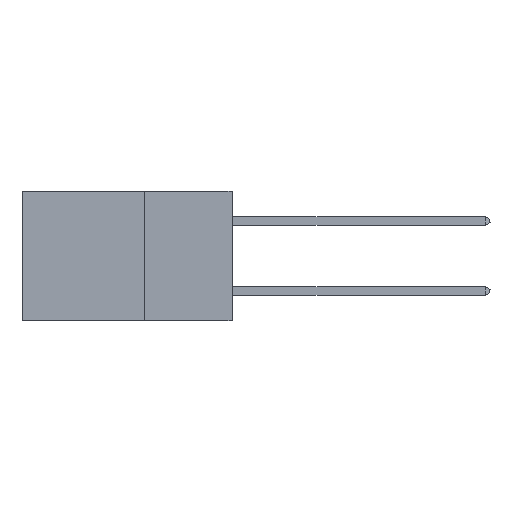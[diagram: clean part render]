
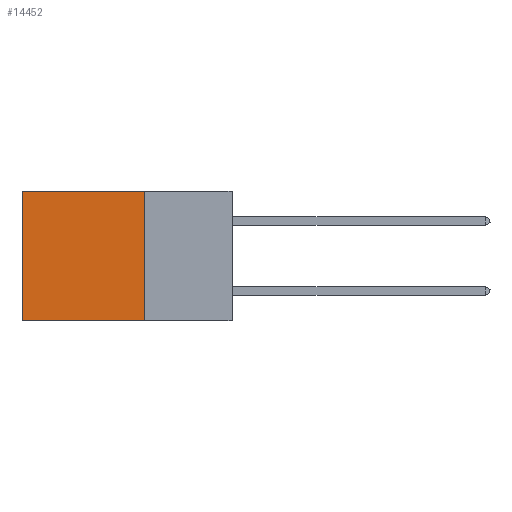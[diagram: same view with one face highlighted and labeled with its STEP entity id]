
A CAD part, left-side view. The second image highlights one B-rep face of the part: STEP entity #14452.
In plain terms, the highlighted planar face has unit normal (-1, 0, 0).
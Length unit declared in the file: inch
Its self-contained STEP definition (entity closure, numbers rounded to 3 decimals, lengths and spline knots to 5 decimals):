
#255 = VERTEX_POINT ( 'NONE', #7116 ) ;
#371 = LINE ( 'NONE', #24608, #9482 ) ;
#1425 = PLANE ( 'NONE',  #29148 ) ;
#1525 = ORIENTED_EDGE ( 'NONE', *, *, #15686, .F. ) ;
#3325 = CARTESIAN_POINT ( 'NONE',  ( 0.2875, 0.25, 0. ) ) ;
#4008 = DIRECTION ( 'NONE',  ( 0., 0., -1. ) ) ;
#5165 = CARTESIAN_POINT ( 'NONE',  ( 0.2875, 0.25, 0. ) ) ;
#5299 = VERTEX_POINT ( 'NONE', #12848 ) ;
#6133 = ORIENTED_EDGE ( 'NONE', *, *, #20132, .T. ) ;
#6477 = CARTESIAN_POINT ( 'NONE',  ( 0.2875, 0.25, -0.37 ) ) ;
#7116 = CARTESIAN_POINT ( 'NONE',  ( 0.2875, 0.25, 0. ) ) ;
#7707 = VERTEX_POINT ( 'NONE', #6477 ) ;
#7900 = DIRECTION ( 'NONE',  ( 0., 0., -1. ) ) ;
#8041 = DIRECTION ( 'NONE',  ( 0., 0., -1. ) ) ;
#8092 = ORIENTED_EDGE ( 'NONE', *, *, #29874, .F. ) ;
#9482 = VECTOR ( 'NONE', #32164, 39.37008 ) ;
#11299 = CARTESIAN_POINT ( 'NONE',  ( 0.2875, 0.6, -0.37 ) ) ;
#12848 = CARTESIAN_POINT ( 'NONE',  ( 0.2875, 0.6, 0. ) ) ;
#14452 = ADVANCED_FACE ( 'NONE', ( #27879 ), #1425, .F. ) ;
#15686 = EDGE_CURVE ( 'NONE', #7707, #18472, #371, .T. ) ;
#18472 = VERTEX_POINT ( 'NONE', #11299 ) ;
#19187 = DIRECTION ( 'NONE',  ( 1., 0., 0. ) ) ;
#20132 = EDGE_CURVE ( 'NONE', #5299, #18472, #22760, .T. ) ;
#20429 = LINE ( 'NONE', #3325, #23227 ) ;
#20488 = VECTOR ( 'NONE', #7900, 39.37008 ) ;
#20841 = CARTESIAN_POINT ( 'NONE',  ( 0.2875, 0.6, 0. ) ) ;
#21646 = ORIENTED_EDGE ( 'NONE', *, *, #30432, .T. ) ;
#22760 = LINE ( 'NONE', #20841, #24729 ) ;
#23227 = VECTOR ( 'NONE', #23855, 39.37008 ) ;
#23855 = DIRECTION ( 'NONE',  ( 0., 1., 0. ) ) ;
#24608 = CARTESIAN_POINT ( 'NONE',  ( 0.2875, 0.25, -0.37 ) ) ;
#24729 = VECTOR ( 'NONE', #8041, 39.37008 ) ;
#26749 = CARTESIAN_POINT ( 'NONE',  ( 0.2875, 0.25, 0. ) ) ;
#27879 = FACE_OUTER_BOUND ( 'NONE', #31579, .T. ) ;
#29148 = AXIS2_PLACEMENT_3D ( 'NONE', #26749, #19187, #4008 ) ;
#29874 = EDGE_CURVE ( 'NONE', #255, #7707, #30440, .T. ) ;
#30432 = EDGE_CURVE ( 'NONE', #255, #5299, #20429, .T. ) ;
#30440 = LINE ( 'NONE', #5165, #20488 ) ;
#31579 = EDGE_LOOP ( 'NONE', ( #6133, #1525, #8092, #21646 ) ) ;
#32164 = DIRECTION ( 'NONE',  ( 0., 1., 0. ) ) ;
